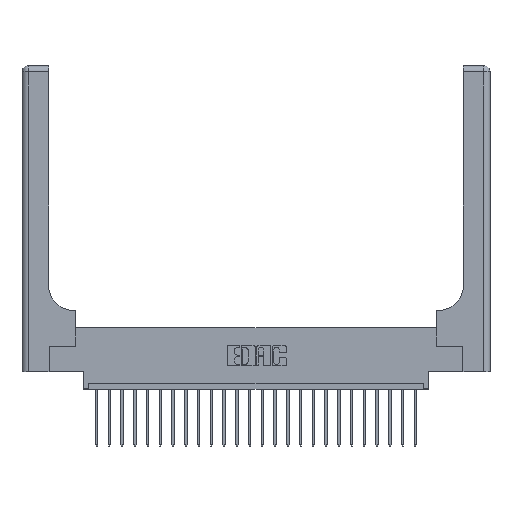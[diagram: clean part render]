
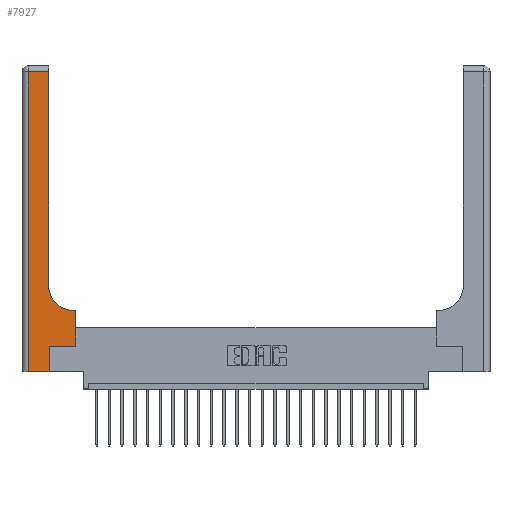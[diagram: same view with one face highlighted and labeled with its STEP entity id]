
A CAD part, top view. The second image highlights one B-rep face of the part: STEP entity #7927.
In plain terms, the highlighted planar face has unit normal (0, 0, 1).
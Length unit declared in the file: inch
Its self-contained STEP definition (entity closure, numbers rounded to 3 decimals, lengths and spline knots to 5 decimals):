
#685 = CARTESIAN_POINT ( 'NONE',  ( 0.528, 0.25, 0.37 ) ) ;
#925 = CARTESIAN_POINT ( 'NONE',  ( 0.51, 0.85, 0.37 ) ) ;
#1080 = LINE ( 'NONE', #8448, #22662 ) ;
#1171 = DIRECTION ( 'NONE',  ( 1., 0., 0. ) ) ;
#1214 = EDGE_CURVE ( 'NONE', #18538, #21991, #4673, .T. ) ;
#1424 = CARTESIAN_POINT ( 'NONE',  ( 0.265, 0., 0.37 ) ) ;
#1425 = ORIENTED_EDGE ( 'NONE', *, *, #3777, .T. ) ;
#1538 = DIRECTION ( 'NONE',  ( 0., 1., 0. ) ) ;
#1685 = CARTESIAN_POINT ( 'NONE',  ( 0., 3., 0.37 ) ) ;
#1876 = ORIENTED_EDGE ( 'NONE', *, *, #3947, .T. ) ;
#2084 = LINE ( 'NONE', #13237, #7505 ) ;
#2120 = VERTEX_POINT ( 'NONE', #17100 ) ;
#2653 = VERTEX_POINT ( 'NONE', #5610 ) ;
#3013 = LINE ( 'NONE', #3142, #8560 ) ;
#3142 = CARTESIAN_POINT ( 'NONE',  ( 0.26, 0.6, 0.37 ) ) ;
#3231 = VERTEX_POINT ( 'NONE', #19430 ) ;
#3502 = LINE ( 'NONE', #18293, #22242 ) ;
#3518 = FACE_OUTER_BOUND ( 'NONE', #9793, .T. ) ;
#3777 = EDGE_CURVE ( 'NONE', #13318, #2120, #3502, .T. ) ;
#3829 = LINE ( 'NONE', #7311, #23862 ) ;
#3947 = EDGE_CURVE ( 'NONE', #13691, #13318, #4021, .T. ) ;
#4021 = CIRCLE ( 'NONE', #22259, 0.25 ) ;
#4406 = EDGE_CURVE ( 'NONE', #3231, #9918, #1080, .T. ) ;
#4673 = LINE ( 'NONE', #12303, #6213 ) ;
#4999 = ORIENTED_EDGE ( 'NONE', *, *, #1214, .T. ) ;
#5610 = CARTESIAN_POINT ( 'NONE',  ( 0.528, 0.6, 0.37 ) ) ;
#6213 = VECTOR ( 'NONE', #1171, 39.37008 ) ;
#6298 = LINE ( 'NONE', #19335, #21207 ) ;
#6326 = EDGE_CURVE ( 'NONE', #21991, #2653, #3829, .T. ) ;
#7171 = AXIS2_PLACEMENT_3D ( 'NONE', #1685, #9076, #12826 ) ;
#7311 = CARTESIAN_POINT ( 'NONE',  ( 0.528, 0.25, 0.37 ) ) ;
#7505 = VECTOR ( 'NONE', #13353, 39.37008 ) ;
#7927 = ADVANCED_FACE ( 'NONE', ( #3518 ), #18312, .F. ) ;
#8234 = ORIENTED_EDGE ( 'NONE', *, *, #10029, .T. ) ;
#8448 = CARTESIAN_POINT ( 'NONE',  ( 0., 0., 0.37 ) ) ;
#8560 = VECTOR ( 'NONE', #23822, 39.37008 ) ;
#8975 = CARTESIAN_POINT ( 'NONE',  ( 0.51, 0.6, 0.37 ) ) ;
#9076 = DIRECTION ( 'NONE',  ( 0., 0., -1. ) ) ;
#9147 = DIRECTION ( 'NONE',  ( 0., 0., -1. ) ) ;
#9793 = EDGE_LOOP ( 'NONE', ( #1425, #11039, #15762, #11684, #8234, #4999, #22735, #23591, #1876 ) ) ;
#9918 = VERTEX_POINT ( 'NONE', #23445 ) ;
#10029 = EDGE_CURVE ( 'NONE', #9918, #18538, #20131, .T. ) ;
#11039 = ORIENTED_EDGE ( 'NONE', *, *, #16236, .T. ) ;
#11205 = DIRECTION ( 'NONE',  ( 0., 1., 0. ) ) ;
#11684 = ORIENTED_EDGE ( 'NONE', *, *, #4406, .T. ) ;
#12303 = CARTESIAN_POINT ( 'NONE',  ( 0.265, 0.25, 0.37 ) ) ;
#12826 = DIRECTION ( 'NONE',  ( -1., 0., 0. ) ) ;
#13237 = CARTESIAN_POINT ( 'NONE',  ( 0., 2.94, 0.37 ) ) ;
#13260 = CARTESIAN_POINT ( 'NONE',  ( 0.26, 0.85, 0.37 ) ) ;
#13318 = VERTEX_POINT ( 'NONE', #13260 ) ;
#13353 = DIRECTION ( 'NONE',  ( -1., 0., 0. ) ) ;
#13691 = VERTEX_POINT ( 'NONE', #8975 ) ;
#14596 = CARTESIAN_POINT ( 'NONE',  ( 0.265, 0.25, 0.37 ) ) ;
#15670 = EDGE_CURVE ( 'NONE', #2653, #13691, #3013, .T. ) ;
#15762 = ORIENTED_EDGE ( 'NONE', *, *, #18649, .T. ) ;
#15776 = DIRECTION ( 'NONE',  ( 1., 0., 0. ) ) ;
#16236 = EDGE_CURVE ( 'NONE', #2120, #19317, #2084, .T. ) ;
#16589 = DIRECTION ( 'NONE',  ( 1., 0., 0. ) ) ;
#17100 = CARTESIAN_POINT ( 'NONE',  ( 0.26, 2.94, 0.37 ) ) ;
#17827 = CARTESIAN_POINT ( 'NONE',  ( 0.06, 2.94, 0.37 ) ) ;
#18135 = VECTOR ( 'NONE', #1538, 39.37008 ) ;
#18293 = CARTESIAN_POINT ( 'NONE',  ( 0.26, 3., 0.37 ) ) ;
#18312 = PLANE ( 'NONE',  #7171 ) ;
#18538 = VERTEX_POINT ( 'NONE', #14596 ) ;
#18649 = EDGE_CURVE ( 'NONE', #19317, #3231, #6298, .T. ) ;
#19317 = VERTEX_POINT ( 'NONE', #17827 ) ;
#19335 = CARTESIAN_POINT ( 'NONE',  ( 0.06, 3., 0.37 ) ) ;
#19430 = CARTESIAN_POINT ( 'NONE',  ( 0.06, 0., 0.37 ) ) ;
#20131 = LINE ( 'NONE', #1424, #18135 ) ;
#20922 = DIRECTION ( 'NONE',  ( 0., -1., 0. ) ) ;
#21207 = VECTOR ( 'NONE', #20922, 39.37008 ) ;
#21991 = VERTEX_POINT ( 'NONE', #685 ) ;
#22242 = VECTOR ( 'NONE', #23472, 39.37008 ) ;
#22259 = AXIS2_PLACEMENT_3D ( 'NONE', #925, #9147, #16589 ) ;
#22662 = VECTOR ( 'NONE', #15776, 39.37008 ) ;
#22735 = ORIENTED_EDGE ( 'NONE', *, *, #6326, .T. ) ;
#23445 = CARTESIAN_POINT ( 'NONE',  ( 0.265, 0., 0.37 ) ) ;
#23472 = DIRECTION ( 'NONE',  ( 0., 1., 0. ) ) ;
#23591 = ORIENTED_EDGE ( 'NONE', *, *, #15670, .T. ) ;
#23822 = DIRECTION ( 'NONE',  ( -1., 0., 0. ) ) ;
#23862 = VECTOR ( 'NONE', #11205, 39.37008 ) ;
